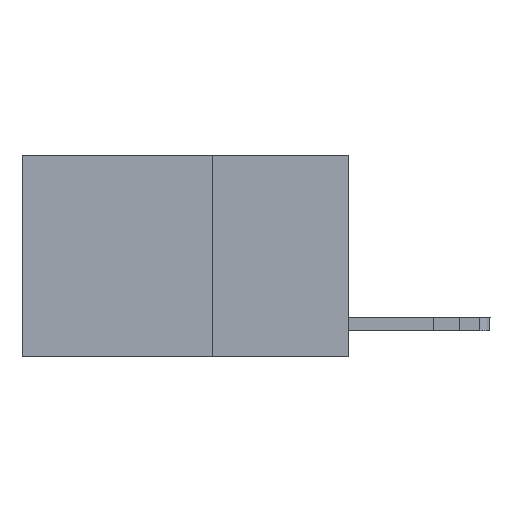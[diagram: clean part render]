
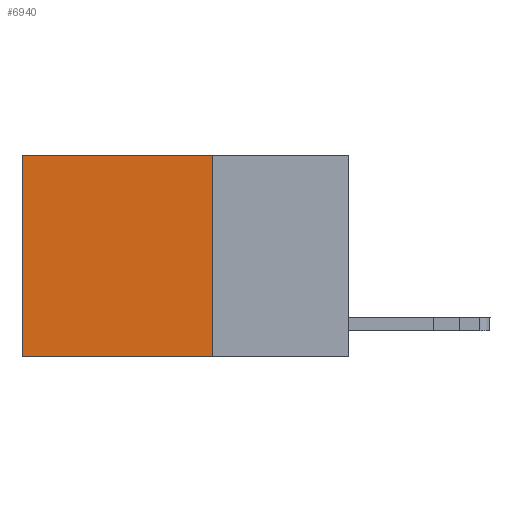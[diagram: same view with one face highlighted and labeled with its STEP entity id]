
A CAD part, left-side view. The second image highlights one B-rep face of the part: STEP entity #6940.
In plain terms, the highlighted planar face has unit normal (-1, 0, 0).
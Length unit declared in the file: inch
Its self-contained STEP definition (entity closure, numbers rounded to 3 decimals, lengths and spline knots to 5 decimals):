
#411 = EDGE_CURVE ( 'NONE', #1549, #5189, #529, .T. ) ;
#529 = LINE ( 'NONE', #11315, #6288 ) ;
#1549 = VERTEX_POINT ( 'NONE', #13052 ) ;
#1736 = VERTEX_POINT ( 'NONE', #3214 ) ;
#1932 = CARTESIAN_POINT ( 'NONE',  ( 0.2625, 0.25, 0. ) ) ;
#2559 = ORIENTED_EDGE ( 'NONE', *, *, #9174, .T. ) ;
#3059 = EDGE_CURVE ( 'NONE', #6253, #5189, #12759, .T. ) ;
#3069 = CARTESIAN_POINT ( 'NONE',  ( 0.2625, 0.6, 0. ) ) ;
#3214 = CARTESIAN_POINT ( 'NONE',  ( 0.2625, 0.25, 0. ) ) ;
#3510 = LINE ( 'NONE', #8781, #10420 ) ;
#3585 = VECTOR ( 'NONE', #5051, 39.37008 ) ;
#4629 = VECTOR ( 'NONE', #10638, 39.37008 ) ;
#4942 = FACE_OUTER_BOUND ( 'NONE', #6664, .T. ) ;
#5051 = DIRECTION ( 'NONE',  ( 0., 1., 0. ) ) ;
#5108 = ORIENTED_EDGE ( 'NONE', *, *, #5405, .F. ) ;
#5189 = VERTEX_POINT ( 'NONE', #11586 ) ;
#5405 = EDGE_CURVE ( 'NONE', #1736, #1549, #3510, .T. ) ;
#6253 = VERTEX_POINT ( 'NONE', #3069 ) ;
#6288 = VECTOR ( 'NONE', #11118, 39.37008 ) ;
#6664 = EDGE_LOOP ( 'NONE', ( #10734, #6966, #5108, #2559 ) ) ;
#6940 = ADVANCED_FACE ( 'NONE', ( #4942 ), #11619, .F. ) ;
#6966 = ORIENTED_EDGE ( 'NONE', *, *, #411, .F. ) ;
#8199 = CARTESIAN_POINT ( 'NONE',  ( 0.2625, 0.25, 0. ) ) ;
#8404 = DIRECTION ( 'NONE',  ( 0., 0., -1. ) ) ;
#8781 = CARTESIAN_POINT ( 'NONE',  ( 0.2625, 0.25, 0. ) ) ;
#9174 = EDGE_CURVE ( 'NONE', #1736, #6253, #10259, .T. ) ;
#9526 = AXIS2_PLACEMENT_3D ( 'NONE', #8199, #10364, #8404 ) ;
#10259 = LINE ( 'NONE', #1932, #3585 ) ;
#10364 = DIRECTION ( 'NONE',  ( 1., 0., 0. ) ) ;
#10420 = VECTOR ( 'NONE', #12978, 39.37008 ) ;
#10638 = DIRECTION ( 'NONE',  ( 0., 0., -1. ) ) ;
#10734 = ORIENTED_EDGE ( 'NONE', *, *, #3059, .T. ) ;
#11118 = DIRECTION ( 'NONE',  ( 0., 1., 0. ) ) ;
#11315 = CARTESIAN_POINT ( 'NONE',  ( 0.2625, 0.25, -0.37 ) ) ;
#11586 = CARTESIAN_POINT ( 'NONE',  ( 0.2625, 0.6, -0.37 ) ) ;
#11619 = PLANE ( 'NONE',  #9526 ) ;
#12759 = LINE ( 'NONE', #13637, #4629 ) ;
#12978 = DIRECTION ( 'NONE',  ( 0., 0., -1. ) ) ;
#13052 = CARTESIAN_POINT ( 'NONE',  ( 0.2625, 0.25, -0.37 ) ) ;
#13637 = CARTESIAN_POINT ( 'NONE',  ( 0.2625, 0.6, 0. ) ) ;
